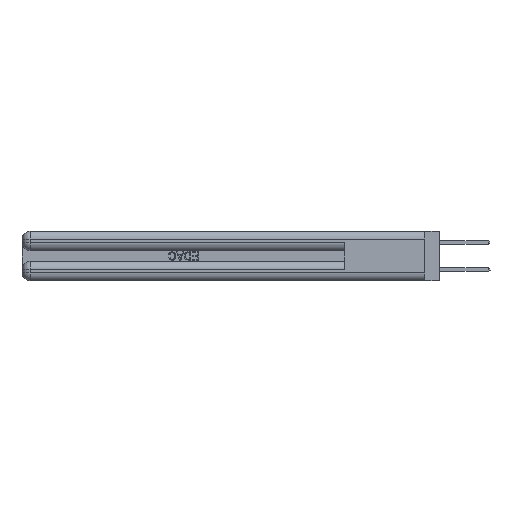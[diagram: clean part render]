
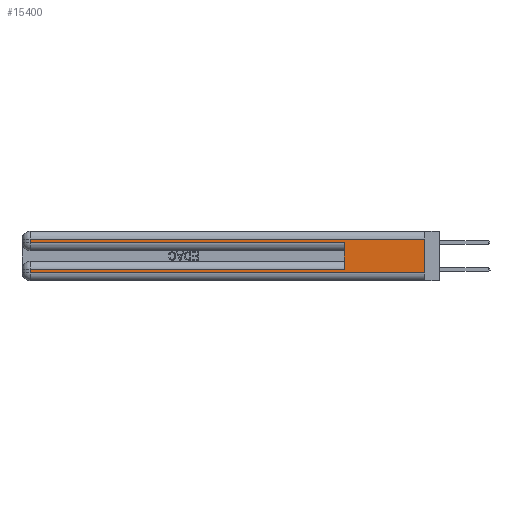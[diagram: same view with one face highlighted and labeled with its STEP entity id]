
A CAD part, left-side view. The second image highlights one B-rep face of the part: STEP entity #15400.
In plain terms, the highlighted planar face has unit normal (-1, 0, 0).
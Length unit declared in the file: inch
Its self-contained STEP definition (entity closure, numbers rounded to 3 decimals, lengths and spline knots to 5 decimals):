
#1282 = DIRECTION ( 'NONE',  ( 0., 1., 0. ) ) ;
#1868 = VECTOR ( 'NONE', #28059, 39.37008 ) ;
#3044 = VERTEX_POINT ( 'NONE', #27298 ) ;
#3319 = DIRECTION ( 'NONE',  ( 0., 0., 1. ) ) ;
#3670 = VECTOR ( 'NONE', #1282, 39.37008 ) ;
#3679 = VECTOR ( 'NONE', #42406, 39.37008 ) ;
#5114 = ORIENTED_EDGE ( 'NONE', *, *, #37819, .T. ) ;
#5588 = VECTOR ( 'NONE', #3319, 39.37008 ) ;
#7840 = VERTEX_POINT ( 'NONE', #26049 ) ;
#8424 = VERTEX_POINT ( 'NONE', #36966 ) ;
#9915 = VECTOR ( 'NONE', #13376, 39.37008 ) ;
#11705 = VECTOR ( 'NONE', #43787, 39.37008 ) ;
#12902 = CARTESIAN_POINT ( 'NONE',  ( 0., 2.94, 0.37 ) ) ;
#13376 = DIRECTION ( 'NONE',  ( 0., -1., 0. ) ) ;
#13409 = CARTESIAN_POINT ( 'NONE',  ( 0., 2.94, 0.37 ) ) ;
#13699 = ORIENTED_EDGE ( 'NONE', *, *, #17546, .T. ) ;
#15176 = CARTESIAN_POINT ( 'NONE',  ( 0., 0., 0.37 ) ) ;
#15281 = LINE ( 'NONE', #39358, #5588 ) ;
#15400 = ADVANCED_FACE ( 'NONE', ( #34491 ), #33232, .F. ) ;
#15798 = ORIENTED_EDGE ( 'NONE', *, *, #32413, .F. ) ;
#16855 = EDGE_CURVE ( 'NONE', #8424, #41300, #41577, .T. ) ;
#17546 = EDGE_CURVE ( 'NONE', #8424, #35495, #21887, .T. ) ;
#17582 = LINE ( 'NONE', #12902, #27231 ) ;
#18447 = LINE ( 'NONE', #38579, #9915 ) ;
#18838 = DIRECTION ( 'NONE',  ( 0., 0., -1. ) ) ;
#19343 = CARTESIAN_POINT ( 'NONE',  ( 0., 0., 0.06 ) ) ;
#19621 = LINE ( 'NONE', #13409, #37617 ) ;
#20802 = CARTESIAN_POINT ( 'NONE',  ( 0., 2.94, 0.06 ) ) ;
#20869 = ORIENTED_EDGE ( 'NONE', *, *, #16855, .F. ) ;
#21344 = EDGE_CURVE ( 'NONE', #35495, #3044, #17582, .T. ) ;
#21887 = LINE ( 'NONE', #23078, #3670 ) ;
#22180 = CARTESIAN_POINT ( 'NONE',  ( 0., 0., 0.37 ) ) ;
#22367 = LINE ( 'NONE', #38820, #1868 ) ;
#23078 = CARTESIAN_POINT ( 'NONE',  ( 0., 0., 0.31 ) ) ;
#23225 = ORIENTED_EDGE ( 'NONE', *, *, #36044, .T. ) ;
#23633 = ORIENTED_EDGE ( 'NONE', *, *, #21344, .T. ) ;
#24374 = DIRECTION ( 'NONE',  ( 0., 0., -1. ) ) ;
#24479 = EDGE_CURVE ( 'NONE', #3044, #7840, #18447, .T. ) ;
#25324 = LINE ( 'NONE', #31678, #3679 ) ;
#25782 = VERTEX_POINT ( 'NONE', #35894 ) ;
#26049 = CARTESIAN_POINT ( 'NONE',  ( 0., 0.6, 0.285 ) ) ;
#27231 = VECTOR ( 'NONE', #38112, 39.37008 ) ;
#27298 = CARTESIAN_POINT ( 'NONE',  ( 0., 2.94, 0.285 ) ) ;
#27594 = EDGE_LOOP ( 'NONE', ( #20869, #13699, #23633, #36542, #15798, #5114, #23225, #37393 ) ) ;
#28059 = DIRECTION ( 'NONE',  ( 0., 1., 0. ) ) ;
#29722 = CARTESIAN_POINT ( 'NONE',  ( 0., 2.94, 0.085 ) ) ;
#30941 = VERTEX_POINT ( 'NONE', #20802 ) ;
#31678 = CARTESIAN_POINT ( 'NONE',  ( 0., 0., 0.06 ) ) ;
#32413 = EDGE_CURVE ( 'NONE', #25782, #7840, #15281, .T. ) ;
#33232 = PLANE ( 'NONE',  #40542 ) ;
#34491 = FACE_OUTER_BOUND ( 'NONE', #27594, .T. ) ;
#35495 = VERTEX_POINT ( 'NONE', #35710 ) ;
#35710 = CARTESIAN_POINT ( 'NONE',  ( 0., 2.94, 0.31 ) ) ;
#35894 = CARTESIAN_POINT ( 'NONE',  ( 0., 0.6, 0.085 ) ) ;
#36044 = EDGE_CURVE ( 'NONE', #44729, #30941, #19621, .T. ) ;
#36542 = ORIENTED_EDGE ( 'NONE', *, *, #24479, .T. ) ;
#36966 = CARTESIAN_POINT ( 'NONE',  ( 0., 0., 0.31 ) ) ;
#37393 = ORIENTED_EDGE ( 'NONE', *, *, #43876, .T. ) ;
#37617 = VECTOR ( 'NONE', #24374, 39.37008 ) ;
#37819 = EDGE_CURVE ( 'NONE', #25782, #44729, #22367, .T. ) ;
#38112 = DIRECTION ( 'NONE',  ( 0., 0., -1. ) ) ;
#38579 = CARTESIAN_POINT ( 'NONE',  ( 0., 0., 0.285 ) ) ;
#38820 = CARTESIAN_POINT ( 'NONE',  ( 0., 0., 0.085 ) ) ;
#39358 = CARTESIAN_POINT ( 'NONE',  ( 0., 0.6, 0.145 ) ) ;
#40359 = DIRECTION ( 'NONE',  ( 1., 0., 0. ) ) ;
#40542 = AXIS2_PLACEMENT_3D ( 'NONE', #15176, #40359, #18838 ) ;
#41300 = VERTEX_POINT ( 'NONE', #19343 ) ;
#41577 = LINE ( 'NONE', #22180, #11705 ) ;
#42406 = DIRECTION ( 'NONE',  ( 0., -1., 0. ) ) ;
#43787 = DIRECTION ( 'NONE',  ( 0., 0., -1. ) ) ;
#43876 = EDGE_CURVE ( 'NONE', #30941, #41300, #25324, .T. ) ;
#44729 = VERTEX_POINT ( 'NONE', #29722 ) ;
